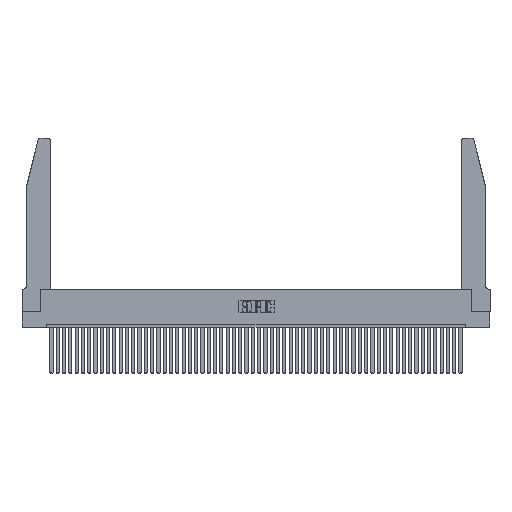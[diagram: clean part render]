
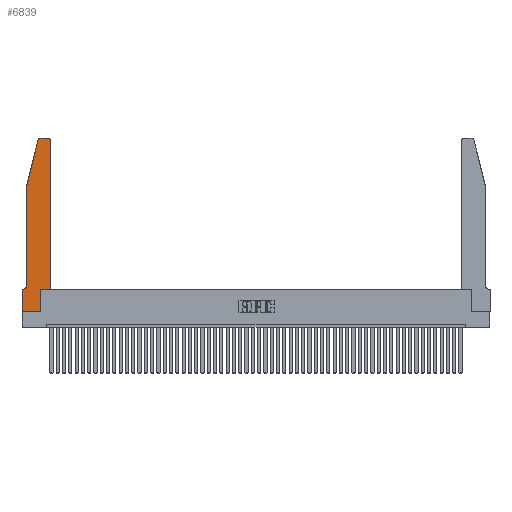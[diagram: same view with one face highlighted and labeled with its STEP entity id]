
A CAD part, top view. The second image highlights one B-rep face of the part: STEP entity #6839.
In plain terms, the highlighted planar face has unit normal (0, 0, 1).
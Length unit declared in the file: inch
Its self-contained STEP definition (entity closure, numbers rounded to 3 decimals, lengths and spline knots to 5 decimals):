
#22 = EDGE_CURVE ( 'NONE', #45424, #4912, #46495, .T. ) ;
#121 = CARTESIAN_POINT ( 'NONE',  ( 0.0755, 2., 0.37 ) ) ;
#532 = DIRECTION ( 'NONE',  ( 0., 0., -1. ) ) ;
#1691 = LINE ( 'NONE', #121, #7291 ) ;
#3277 = CARTESIAN_POINT ( 'NONE',  ( 0.2865, 0.35, 0.37 ) ) ;
#3282 = VECTOR ( 'NONE', #11136, 39.37008 ) ;
#3379 = EDGE_CURVE ( 'NONE', #43072, #4936, #15602, .T. ) ;
#4912 = VERTEX_POINT ( 'NONE', #3277 ) ;
#4919 = VERTEX_POINT ( 'NONE', #14985 ) ;
#4936 = VERTEX_POINT ( 'NONE', #34004 ) ;
#5254 = VERTEX_POINT ( 'NONE', #40897 ) ;
#6287 = DIRECTION ( 'NONE',  ( -1., 0., 0. ) ) ;
#6493 = ORIENTED_EDGE ( 'NONE', *, *, #39969, .T. ) ;
#6839 = ADVANCED_FACE ( 'NONE', ( #42351 ), #29075, .T. ) ;
#7291 = VECTOR ( 'NONE', #8018, 39.37008 ) ;
#7740 = CARTESIAN_POINT ( 'NONE',  ( 0.4505, 0.35, 0.37 ) ) ;
#8018 = DIRECTION ( 'NONE',  ( -0.239, -0.971, 0. ) ) ;
#8434 = AXIS2_PLACEMENT_3D ( 'NONE', #16030, #532, #16349 ) ;
#8686 = ORIENTED_EDGE ( 'NONE', *, *, #49989, .T. ) ;
#9148 = CARTESIAN_POINT ( 'NONE',  ( 0.0755, 0.42, 0.37 ) ) ;
#10297 = VECTOR ( 'NONE', #50881, 39.37008 ) ;
#10621 = ORIENTED_EDGE ( 'NONE', *, *, #3379, .T. ) ;
#10818 = ORIENTED_EDGE ( 'NONE', *, *, #50344, .T. ) ;
#11136 = DIRECTION ( 'NONE',  ( 1., 0., 0. ) ) ;
#12103 = CIRCLE ( 'NONE', #8434, 0.07 ) ;
#13468 = EDGE_CURVE ( 'NONE', #4936, #23336, #26480, .T. ) ;
#14085 = DIRECTION ( 'NONE',  ( 0., 0., 1. ) ) ;
#14306 = CARTESIAN_POINT ( 'NONE',  ( 0., 0.35, 0.37 ) ) ;
#14985 = CARTESIAN_POINT ( 'NONE',  ( 0., 0., 0.37 ) ) ;
#15602 = LINE ( 'NONE', #34273, #19313 ) ;
#16030 = CARTESIAN_POINT ( 'NONE',  ( 0.0055, 0.42, 0.37 ) ) ;
#16349 = DIRECTION ( 'NONE',  ( -1., 0., 0. ) ) ;
#16746 = DIRECTION ( 'NONE',  ( -1., 0., 0. ) ) ;
#18922 = EDGE_CURVE ( 'NONE', #45280, #44874, #1691, .T. ) ;
#18984 = VECTOR ( 'NONE', #19754, 39.37008 ) ;
#19313 = VECTOR ( 'NONE', #25806, 39.37008 ) ;
#19350 = CARTESIAN_POINT ( 'NONE',  ( 0.0755, 2., 0.37 ) ) ;
#19442 = ORIENTED_EDGE ( 'NONE', *, *, #45559, .T. ) ;
#19754 = DIRECTION ( 'NONE',  ( 1., 0., 0. ) ) ;
#19911 = CARTESIAN_POINT ( 'NONE',  ( 0.4205, 2.75, 0.37 ) ) ;
#21489 = EDGE_CURVE ( 'NONE', #44874, #40309, #22688, .T. ) ;
#21532 = CARTESIAN_POINT ( 'NONE',  ( 0.284, 2.75, 0.37 ) ) ;
#22264 = ORIENTED_EDGE ( 'NONE', *, *, #21489, .T. ) ;
#22488 = CARTESIAN_POINT ( 'NONE',  ( 0.2605, 2.75, 0.37 ) ) ;
#22688 = LINE ( 'NONE', #19350, #10297 ) ;
#23336 = VERTEX_POINT ( 'NONE', #19911 ) ;
#23835 = CARTESIAN_POINT ( 'NONE',  ( 0.25487, 2.72718, 0.37 ) ) ;
#24145 = VECTOR ( 'NONE', #16746, 39.37008 ) ;
#24787 = CARTESIAN_POINT ( 'NONE',  ( 0.4505, 0.35, 0.37 ) ) ;
#24809 = AXIS2_PLACEMENT_3D ( 'NONE', #33797, #41867, #45988 ) ;
#25806 = DIRECTION ( 'NONE',  ( 0., 1., 0. ) ) ;
#25844 = DIRECTION ( 'NONE',  ( 1., 0., 0. ) ) ;
#25885 = ORIENTED_EDGE ( 'NONE', *, *, #13468, .T. ) ;
#25915 = ORIENTED_EDGE ( 'NONE', *, *, #22, .T. ) ;
#26007 = CARTESIAN_POINT ( 'NONE',  ( 0.4205, 2.72, 0.37 ) ) ;
#26100 = LINE ( 'NONE', #50416, #3282 ) ;
#26313 = ORIENTED_EDGE ( 'NONE', *, *, #18922, .T. ) ;
#26480 = CIRCLE ( 'NONE', #44363, 0.03 ) ;
#27391 = VECTOR ( 'NONE', #44250, 39.37008 ) ;
#27957 = EDGE_CURVE ( 'NONE', #40309, #5254, #12103, .T. ) ;
#28223 = CARTESIAN_POINT ( 'NONE',  ( 0.0755, 2., 0.37 ) ) ;
#28770 = CARTESIAN_POINT ( 'NONE',  ( 0.2865, 0.35, 0.37 ) ) ;
#29075 = PLANE ( 'NONE',  #35982 ) ;
#29237 = VECTOR ( 'NONE', #45250, 39.37008 ) ;
#29273 = EDGE_LOOP ( 'NONE', ( #10818, #19442, #26313, #22264, #48199, #38482, #48087, #8686, #25915, #6493, #10621, #25885 ) ) ;
#29615 = CARTESIAN_POINT ( 'NONE',  ( 0., 0.35, 0.37 ) ) ;
#32762 = CARTESIAN_POINT ( 'NONE',  ( 0.2865, 0., 0.37 ) ) ;
#33049 = DIRECTION ( 'NONE',  ( 1., 0., 0. ) ) ;
#33797 = CARTESIAN_POINT ( 'NONE',  ( 0.284, 2.72, 0.37 ) ) ;
#34004 = CARTESIAN_POINT ( 'NONE',  ( 0.4505, 2.72, 0.37 ) ) ;
#34273 = CARTESIAN_POINT ( 'NONE',  ( 0.4505, 0.35, 0.37 ) ) ;
#35982 = AXIS2_PLACEMENT_3D ( 'NONE', #29615, #37192, #33049 ) ;
#36053 = LINE ( 'NONE', #38475, #29237 ) ;
#36151 = VERTEX_POINT ( 'NONE', #14306 ) ;
#36309 = EDGE_CURVE ( 'NONE', #36151, #4919, #36053, .T. ) ;
#37192 = DIRECTION ( 'NONE',  ( 0., 0., 1. ) ) ;
#37716 = LINE ( 'NONE', #44830, #24145 ) ;
#38475 = CARTESIAN_POINT ( 'NONE',  ( 0., 0., 0.37 ) ) ;
#38482 = ORIENTED_EDGE ( 'NONE', *, *, #43749, .T. ) ;
#39940 = LINE ( 'NONE', #7740, #18984 ) ;
#39969 = EDGE_CURVE ( 'NONE', #4912, #43072, #39940, .T. ) ;
#40309 = VERTEX_POINT ( 'NONE', #9148 ) ;
#40897 = CARTESIAN_POINT ( 'NONE',  ( 0.0055, 0.35, 0.37 ) ) ;
#41760 = VERTEX_POINT ( 'NONE', #21532 ) ;
#41867 = DIRECTION ( 'NONE',  ( 0., 0., 1. ) ) ;
#42351 = FACE_OUTER_BOUND ( 'NONE', #29273, .T. ) ;
#43072 = VERTEX_POINT ( 'NONE', #24787 ) ;
#43749 = EDGE_CURVE ( 'NONE', #5254, #36151, #37716, .T. ) ;
#44250 = DIRECTION ( 'NONE',  ( 0., 1., 0. ) ) ;
#44363 = AXIS2_PLACEMENT_3D ( 'NONE', #26007, #14085, #25844 ) ;
#44830 = CARTESIAN_POINT ( 'NONE',  ( 0.0755, 0.35, 0.37 ) ) ;
#44874 = VERTEX_POINT ( 'NONE', #28223 ) ;
#45250 = DIRECTION ( 'NONE',  ( 0., -1., 0. ) ) ;
#45280 = VERTEX_POINT ( 'NONE', #23835 ) ;
#45424 = VERTEX_POINT ( 'NONE', #32762 ) ;
#45559 = EDGE_CURVE ( 'NONE', #41760, #45280, #46232, .T. ) ;
#45988 = DIRECTION ( 'NONE',  ( 1., 0., 0. ) ) ;
#46232 = CIRCLE ( 'NONE', #24809, 0.03 ) ;
#46398 = VECTOR ( 'NONE', #6287, 39.37008 ) ;
#46495 = LINE ( 'NONE', #28770, #27391 ) ;
#47617 = LINE ( 'NONE', #22488, #46398 ) ;
#48087 = ORIENTED_EDGE ( 'NONE', *, *, #36309, .T. ) ;
#48199 = ORIENTED_EDGE ( 'NONE', *, *, #27957, .T. ) ;
#49989 = EDGE_CURVE ( 'NONE', #4919, #45424, #26100, .T. ) ;
#50344 = EDGE_CURVE ( 'NONE', #23336, #41760, #47617, .T. ) ;
#50416 = CARTESIAN_POINT ( 'NONE',  ( 0., 0., 0.37 ) ) ;
#50881 = DIRECTION ( 'NONE',  ( 0., -1., 0. ) ) ;
